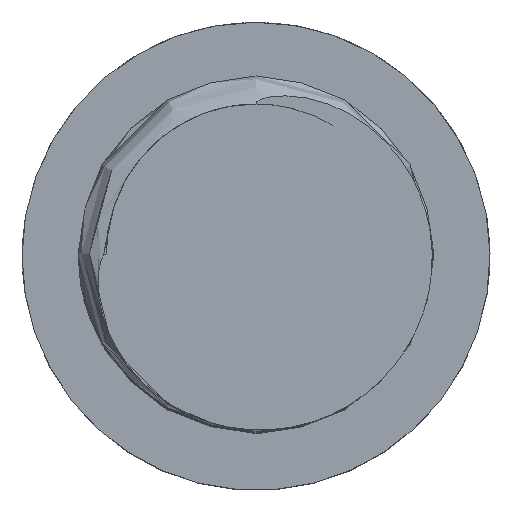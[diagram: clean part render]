
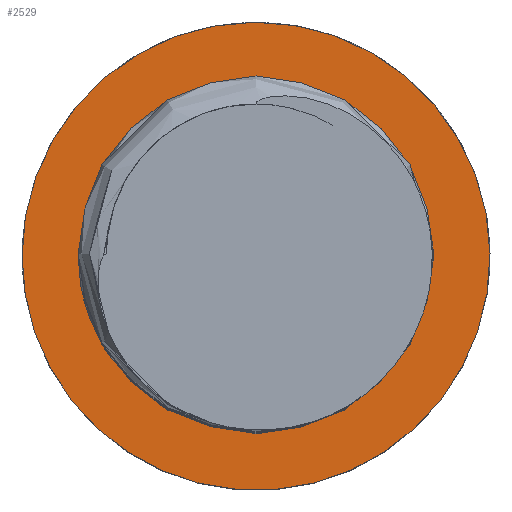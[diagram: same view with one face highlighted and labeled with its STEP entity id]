
A CAD part, top view. The second image highlights one B-rep face of the part: STEP entity #2529.
In plain terms, the highlighted planar face has unit normal (0, 0, 1).
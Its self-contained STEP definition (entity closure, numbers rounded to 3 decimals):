
#180 = DIRECTION ( 'NONE',  ( 0., 0., -1. ) ) ;
#196 = AXIS2_PLACEMENT_3D ( 'NONE', #2925, #224, #3575 ) ;
#217 = AXIS2_PLACEMENT_3D ( 'NONE', #238, #2606, #582 ) ;
#224 = DIRECTION ( 'NONE',  ( 0., 0., -1. ) ) ;
#238 = CARTESIAN_POINT ( 'NONE',  ( 0., 0., 0. ) ) ;
#555 = ORIENTED_EDGE ( 'NONE', *, *, #2238, .T. ) ;
#563 = ORIENTED_EDGE ( 'NONE', *, *, #2554, .F. ) ;
#582 = DIRECTION ( 'NONE',  ( -1., 0., 0. ) ) ;
#624 = CARTESIAN_POINT ( 'NONE',  ( -5., 0., 0. ) ) ;
#731 = AXIS2_PLACEMENT_3D ( 'NONE', #2208, #180, #2552 ) ;
#1657 = EDGE_LOOP ( 'NONE', ( #555 ) ) ;
#1743 = VERTEX_POINT ( 'NONE', #624 ) ;
#2190 = EDGE_LOOP ( 'NONE', ( #563 ) ) ;
#2208 = CARTESIAN_POINT ( 'NONE',  ( 0., 0., 0. ) ) ;
#2238 = EDGE_CURVE ( 'NONE', #1743, #1743, #4223, .T. ) ;
#2529 = ADVANCED_FACE ( 'NONE', ( #4062, #4046 ), #3251, .F. ) ;
#2552 = DIRECTION ( 'NONE',  ( -1., 0., 0. ) ) ;
#2554 = EDGE_CURVE ( 'NONE', #3872, #3872, #4094, .T. ) ;
#2606 = DIRECTION ( 'NONE',  ( 0., 0., -1. ) ) ;
#2925 = CARTESIAN_POINT ( 'NONE',  ( 0., 0., 0. ) ) ;
#3251 = PLANE ( 'NONE',  #196 ) ;
#3575 = DIRECTION ( 'NONE',  ( -1., 0., 0. ) ) ;
#3615 = CARTESIAN_POINT ( 'NONE',  ( -12.5, 0., 0. ) ) ;
#3872 = VERTEX_POINT ( 'NONE', #3615 ) ;
#4046 = FACE_OUTER_BOUND ( 'NONE', #2190, .T. ) ;
#4062 = FACE_BOUND ( 'NONE', #1657, .T. ) ;
#4094 = CIRCLE ( 'NONE', #217, 12.5 ) ;
#4223 = CIRCLE ( 'NONE', #731, 5. ) ;
